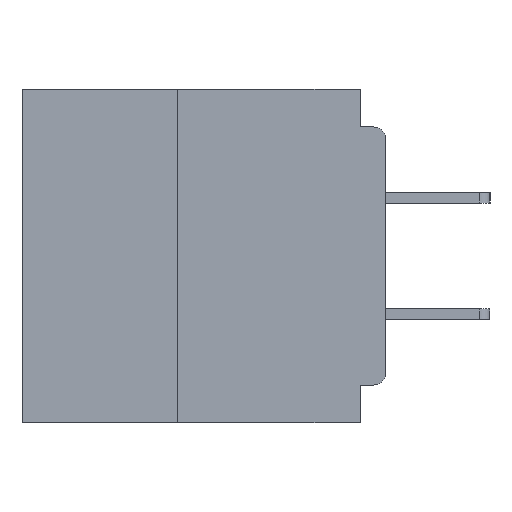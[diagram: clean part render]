
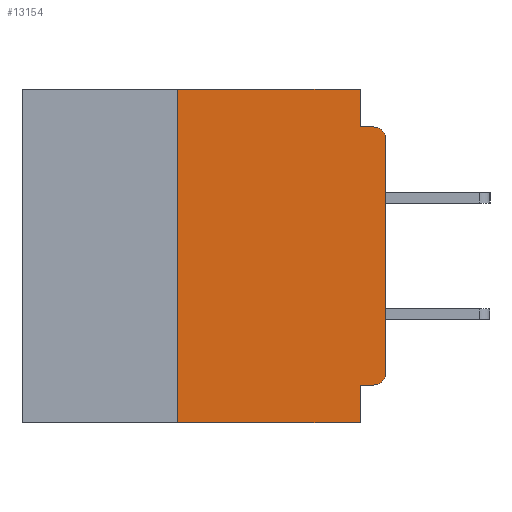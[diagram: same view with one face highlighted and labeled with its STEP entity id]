
A CAD part, left-side view. The second image highlights one B-rep face of the part: STEP entity #13154.
In plain terms, the highlighted planar face has unit normal (-1, 0, 0).
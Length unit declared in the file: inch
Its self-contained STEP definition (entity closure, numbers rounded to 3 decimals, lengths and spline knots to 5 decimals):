
#734 = FACE_OUTER_BOUND ( 'NONE', #17376, .T. ) ;
#1012 = CARTESIAN_POINT ( 'NONE',  ( 0., 0.031, -0.355 ) ) ;
#1626 = CARTESIAN_POINT ( 'NONE',  ( 0., 0.25, -0.4 ) ) ;
#2975 = ORIENTED_EDGE ( 'NONE', *, *, #9198, .T. ) ;
#3003 = CARTESIAN_POINT ( 'NONE',  ( 0., 0.437, -0.4 ) ) ;
#4948 = LINE ( 'NONE', #17255, #55716 ) ;
#6235 = ORIENTED_EDGE ( 'NONE', *, *, #19747, .T. ) ;
#6398 = EDGE_CURVE ( 'NONE', #41385, #38251, #13733, .T. ) ;
#7452 = LINE ( 'NONE', #33215, #61220 ) ;
#9198 = EDGE_CURVE ( 'NONE', #27589, #21269, #42018, .T. ) ;
#9331 = ORIENTED_EDGE ( 'NONE', *, *, #54420, .F. ) ;
#9440 = EDGE_CURVE ( 'NONE', #61823, #21269, #42756, .T. ) ;
#9544 = CARTESIAN_POINT ( 'NONE',  ( 0., 0.031, -0.4 ) ) ;
#10098 = CARTESIAN_POINT ( 'NONE',  ( 0., 0.25, -0.4 ) ) ;
#11198 = DIRECTION ( 'NONE',  ( 0., 1., 0. ) ) ;
#12099 = EDGE_CURVE ( 'NONE', #51329, #29750, #33253, .T. ) ;
#13154 = ADVANCED_FACE ( 'NONE', ( #734 ), #42529, .F. ) ;
#13733 = LINE ( 'NONE', #43592, #51323 ) ;
#13927 = CARTESIAN_POINT ( 'NONE',  ( 0., 0.015, -0.06 ) ) ;
#13933 = ORIENTED_EDGE ( 'NONE', *, *, #12099, .T. ) ;
#14974 = ORIENTED_EDGE ( 'NONE', *, *, #16618, .F. ) ;
#15036 = VECTOR ( 'NONE', #45474, 39.37008 ) ;
#15630 = DIRECTION ( 'NONE',  ( 0., -1., 0. ) ) ;
#15951 = ORIENTED_EDGE ( 'NONE', *, *, #54362, .F. ) ;
#16618 = EDGE_CURVE ( 'NONE', #47591, #17530, #4948, .T. ) ;
#17100 = EDGE_CURVE ( 'NONE', #29750, #27589, #41128, .T. ) ;
#17255 = CARTESIAN_POINT ( 'NONE',  ( 0., 0.031, -0.4 ) ) ;
#17376 = EDGE_LOOP ( 'NONE', ( #19813, #2975, #60852, #57867, #51970, #9331, #6235, #14974, #15951, #13933 ) ) ;
#17530 = VERTEX_POINT ( 'NONE', #9544 ) ;
#18099 = CARTESIAN_POINT ( 'NONE',  ( 0., 0.437, 0. ) ) ;
#18876 = DIRECTION ( 'NONE',  ( 0., 0., -1. ) ) ;
#19057 = DIRECTION ( 'NONE',  ( -1., 0., 0. ) ) ;
#19675 = CARTESIAN_POINT ( 'NONE',  ( 0., 0.031, 0. ) ) ;
#19747 = EDGE_CURVE ( 'NONE', #59338, #17530, #28582, .T. ) ;
#19813 = ORIENTED_EDGE ( 'NONE', *, *, #17100, .T. ) ;
#20052 = AXIS2_PLACEMENT_3D ( 'NONE', #18099, #52359, #23057 ) ;
#21077 = CARTESIAN_POINT ( 'NONE',  ( 0., 0., 0. ) ) ;
#21269 = VERTEX_POINT ( 'NONE', #34062 ) ;
#21341 = VECTOR ( 'NONE', #15630, 39.37008 ) ;
#23057 = DIRECTION ( 'NONE',  ( 0., 0., -1. ) ) ;
#27066 = VECTOR ( 'NONE', #56985, 39.37008 ) ;
#27589 = VERTEX_POINT ( 'NONE', #45810 ) ;
#28582 = LINE ( 'NONE', #3003, #27066 ) ;
#29750 = VERTEX_POINT ( 'NONE', #47683 ) ;
#33215 = CARTESIAN_POINT ( 'NONE',  ( 0., 0.031, 0. ) ) ;
#33253 = CIRCLE ( 'NONE', #47887, 0.015 ) ;
#34062 = CARTESIAN_POINT ( 'NONE',  ( 0., 0.015, -0.045 ) ) ;
#34469 = CARTESIAN_POINT ( 'NONE',  ( 0., 0.031, -0.045 ) ) ;
#38251 = VERTEX_POINT ( 'NONE', #19675 ) ;
#39380 = LINE ( 'NONE', #1626, #50853 ) ;
#40399 = AXIS2_PLACEMENT_3D ( 'NONE', #13927, #48191, #18876 ) ;
#40916 = VECTOR ( 'NONE', #11198, 39.37008 ) ;
#41106 = CARTESIAN_POINT ( 'NONE',  ( 0., 0.25, 0. ) ) ;
#41128 = LINE ( 'NONE', #21077, #15036 ) ;
#41385 = VERTEX_POINT ( 'NONE', #41106 ) ;
#42018 = CIRCLE ( 'NONE', #40399, 0.015 ) ;
#42529 = PLANE ( 'NONE',  #20052 ) ;
#42756 = LINE ( 'NONE', #49883, #21341 ) ;
#43592 = CARTESIAN_POINT ( 'NONE',  ( 0., 0.437, 0. ) ) ;
#44705 = CARTESIAN_POINT ( 'NONE',  ( 0., 0.015, -0.355 ) ) ;
#45474 = DIRECTION ( 'NONE',  ( 0., 0., 1. ) ) ;
#45515 = LINE ( 'NONE', #50463, #40916 ) ;
#45810 = CARTESIAN_POINT ( 'NONE',  ( 0., 0., -0.06 ) ) ;
#45974 = DIRECTION ( 'NONE',  ( 0., 0., 1. ) ) ;
#47591 = VERTEX_POINT ( 'NONE', #1012 ) ;
#47683 = CARTESIAN_POINT ( 'NONE',  ( 0., 0., -0.34 ) ) ;
#47887 = AXIS2_PLACEMENT_3D ( 'NONE', #48373, #19057, #53308 ) ;
#48191 = DIRECTION ( 'NONE',  ( -1., 0., 0. ) ) ;
#48373 = CARTESIAN_POINT ( 'NONE',  ( 0., 0.015, -0.34 ) ) ;
#49883 = CARTESIAN_POINT ( 'NONE',  ( 0., 0., -0.045 ) ) ;
#50463 = CARTESIAN_POINT ( 'NONE',  ( 0., 0., -0.355 ) ) ;
#50853 = VECTOR ( 'NONE', #45974, 39.37008 ) ;
#51323 = VECTOR ( 'NONE', #63289, 39.37008 ) ;
#51329 = VERTEX_POINT ( 'NONE', #44705 ) ;
#51510 = DIRECTION ( 'NONE',  ( 0., 0., -1. ) ) ;
#51970 = ORIENTED_EDGE ( 'NONE', *, *, #6398, .F. ) ;
#52359 = DIRECTION ( 'NONE',  ( 1., 0., 0. ) ) ;
#52735 = DIRECTION ( 'NONE',  ( 0., 0., -1. ) ) ;
#53308 = DIRECTION ( 'NONE',  ( 0., 0., -1. ) ) ;
#54362 = EDGE_CURVE ( 'NONE', #51329, #47591, #45515, .T. ) ;
#54420 = EDGE_CURVE ( 'NONE', #59338, #41385, #39380, .T. ) ;
#55716 = VECTOR ( 'NONE', #51510, 39.37008 ) ;
#56985 = DIRECTION ( 'NONE',  ( 0., -1., 0. ) ) ;
#57867 = ORIENTED_EDGE ( 'NONE', *, *, #61650, .F. ) ;
#59338 = VERTEX_POINT ( 'NONE', #10098 ) ;
#60852 = ORIENTED_EDGE ( 'NONE', *, *, #9440, .F. ) ;
#61220 = VECTOR ( 'NONE', #52735, 39.37008 ) ;
#61650 = EDGE_CURVE ( 'NONE', #38251, #61823, #7452, .T. ) ;
#61823 = VERTEX_POINT ( 'NONE', #34469 ) ;
#63289 = DIRECTION ( 'NONE',  ( 0., -1., 0. ) ) ;
